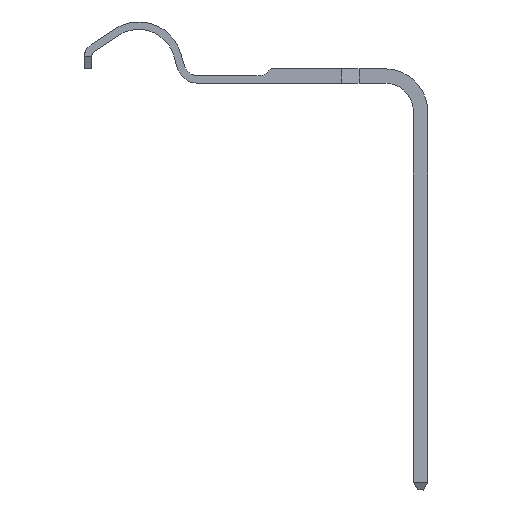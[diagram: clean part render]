
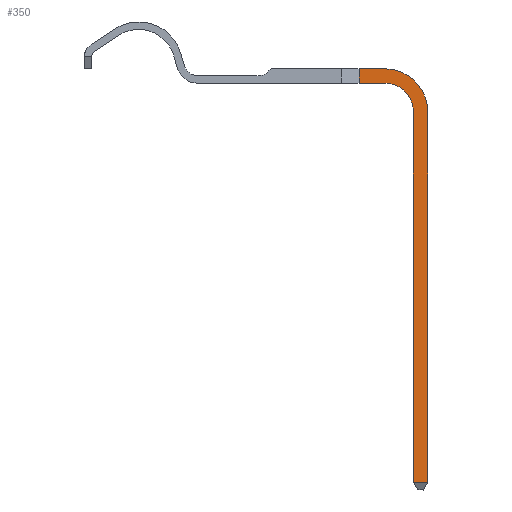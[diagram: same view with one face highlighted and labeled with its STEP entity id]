
A CAD part, left-side view. The second image highlights one B-rep face of the part: STEP entity #350.
In plain terms, the highlighted face is planar.
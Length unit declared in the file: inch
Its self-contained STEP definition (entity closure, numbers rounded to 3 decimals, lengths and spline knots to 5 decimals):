
#196 = VECTOR ( 'NONE', #22878, 39.37008 ) ;
#277 = DIRECTION ( 'NONE',  ( 0., -1., 0. ) ) ;
#350 = ADVANCED_FACE ( 'NONE', ( #4879 ), #11792, .F. ) ;
#1325 = LINE ( 'NONE', #15670, #196 ) ;
#1687 = CARTESIAN_POINT ( 'NONE',  ( 0.65571, -0.0375, 0.0125 ) ) ;
#2143 = VERTEX_POINT ( 'NONE', #17057 ) ;
#2329 = VERTEX_POINT ( 'NONE', #5376 ) ;
#2948 = EDGE_CURVE ( 'NONE', #5791, #10489, #14399, .T. ) ;
#3137 = CARTESIAN_POINT ( 'NONE',  ( 0.70571, -0.0375, 0.0125 ) ) ;
#3449 = ORIENTED_EDGE ( 'NONE', *, *, #2948, .T. ) ;
#4358 = VECTOR ( 'NONE', #14362, 39.37008 ) ;
#4509 = VERTEX_POINT ( 'NONE', #22794 ) ;
#4562 = EDGE_CURVE ( 'NONE', #2143, #18133, #22574, .T. ) ;
#4751 = DIRECTION ( 'NONE',  ( -1., 0., 0. ) ) ;
#4879 = FACE_OUTER_BOUND ( 'NONE', #10164, .T. ) ;
#4985 = CARTESIAN_POINT ( 'NONE',  ( 0.65571, -0.0375, 0.0125 ) ) ;
#5375 = LINE ( 'NONE', #21375, #10362 ) ;
#5376 = CARTESIAN_POINT ( 'NONE',  ( 0.73071, -0.682, 0.0125 ) ) ;
#5493 = ORIENTED_EDGE ( 'NONE', *, *, #16275, .T. ) ;
#5647 = CARTESIAN_POINT ( 'NONE',  ( 0.58021, 0.0375, 0.0125 ) ) ;
#5658 = ORIENTED_EDGE ( 'NONE', *, *, #4562, .T. ) ;
#5791 = VERTEX_POINT ( 'NONE', #21946 ) ;
#5913 = VECTOR ( 'NONE', #18840, 39.37008 ) ;
#7293 = LINE ( 'NONE', #5647, #4358 ) ;
#7792 = CARTESIAN_POINT ( 'NONE',  ( 0.61115, -0.0375, 0.0125 ) ) ;
#8620 = CIRCLE ( 'NONE', #21806, 0.05 ) ;
#8728 = DIRECTION ( 'NONE',  ( -1., 0., 0. ) ) ;
#10026 = DIRECTION ( 'NONE',  ( -1., 0., 0. ) ) ;
#10164 = EDGE_LOOP ( 'NONE', ( #5658, #12287, #5493, #3449, #12918, #16297, #15570, #16956 ) ) ;
#10280 = DIRECTION ( 'NONE',  ( 0., -1., 0. ) ) ;
#10289 = DIRECTION ( 'NONE',  ( 0., 1., 0. ) ) ;
#10362 = VECTOR ( 'NONE', #10289, 39.37008 ) ;
#10489 = VERTEX_POINT ( 'NONE', #21048 ) ;
#11374 = VERTEX_POINT ( 'NONE', #23001 ) ;
#11411 = EDGE_CURVE ( 'NONE', #11746, #2143, #8620, .T. ) ;
#11522 = EDGE_CURVE ( 'NONE', #4509, #11374, #21835, .T. ) ;
#11746 = VERTEX_POINT ( 'NONE', #13752 ) ;
#11792 = PLANE ( 'NONE',  #14464 ) ;
#12040 = DIRECTION ( 'NONE',  ( 0., 0., -1. ) ) ;
#12287 = ORIENTED_EDGE ( 'NONE', *, *, #12516, .T. ) ;
#12516 = EDGE_CURVE ( 'NONE', #18133, #2329, #18405, .T. ) ;
#12918 = ORIENTED_EDGE ( 'NONE', *, *, #22141, .T. ) ;
#13752 = CARTESIAN_POINT ( 'NONE',  ( 0.65571, 0.0125, 0.0125 ) ) ;
#14362 = DIRECTION ( 'NONE',  ( -1., 0., 0. ) ) ;
#14399 = CIRCLE ( 'NONE', #20795, 0.075 ) ;
#14464 = AXIS2_PLACEMENT_3D ( 'NONE', #4985, #12040, #10026 ) ;
#15103 = CARTESIAN_POINT ( 'NONE',  ( 0.70571, -0.682, 0.0125 ) ) ;
#15161 = VECTOR ( 'NONE', #10280, 39.37008 ) ;
#15570 = ORIENTED_EDGE ( 'NONE', *, *, #15770, .T. ) ;
#15670 = CARTESIAN_POINT ( 'NONE',  ( 0.58021, 0.0125, 0.0125 ) ) ;
#15770 = EDGE_CURVE ( 'NONE', #11374, #11746, #1325, .T. ) ;
#16033 = DIRECTION ( 'NONE',  ( 0., 0., -1. ) ) ;
#16275 = EDGE_CURVE ( 'NONE', #2329, #5791, #5375, .T. ) ;
#16297 = ORIENTED_EDGE ( 'NONE', *, *, #11522, .T. ) ;
#16711 = CARTESIAN_POINT ( 'NONE',  ( 0.65571, -0.682, 0.0125 ) ) ;
#16956 = ORIENTED_EDGE ( 'NONE', *, *, #11411, .T. ) ;
#17057 = CARTESIAN_POINT ( 'NONE',  ( 0.70571, -0.0375, 0.0125 ) ) ;
#17218 = VECTOR ( 'NONE', #277, 39.37008 ) ;
#18133 = VERTEX_POINT ( 'NONE', #15103 ) ;
#18405 = LINE ( 'NONE', #16711, #5913 ) ;
#18840 = DIRECTION ( 'NONE',  ( 1., 0., 0. ) ) ;
#20795 = AXIS2_PLACEMENT_3D ( 'NONE', #22643, #20888, #4751 ) ;
#20888 = DIRECTION ( 'NONE',  ( 0., 0., 1. ) ) ;
#21048 = CARTESIAN_POINT ( 'NONE',  ( 0.65571, 0.0375, 0.0125 ) ) ;
#21375 = CARTESIAN_POINT ( 'NONE',  ( 0.73071, -0.0375, 0.0125 ) ) ;
#21806 = AXIS2_PLACEMENT_3D ( 'NONE', #1687, #16033, #8728 ) ;
#21835 = LINE ( 'NONE', #7792, #17218 ) ;
#21946 = CARTESIAN_POINT ( 'NONE',  ( 0.73071, -0.0375, 0.0125 ) ) ;
#22141 = EDGE_CURVE ( 'NONE', #10489, #4509, #7293, .T. ) ;
#22574 = LINE ( 'NONE', #3137, #15161 ) ;
#22643 = CARTESIAN_POINT ( 'NONE',  ( 0.65571, -0.0375, 0.0125 ) ) ;
#22794 = CARTESIAN_POINT ( 'NONE',  ( 0.61115, 0.0375, 0.0125 ) ) ;
#22878 = DIRECTION ( 'NONE',  ( 1., 0., 0. ) ) ;
#23001 = CARTESIAN_POINT ( 'NONE',  ( 0.61115, 0.0125, 0.0125 ) ) ;
